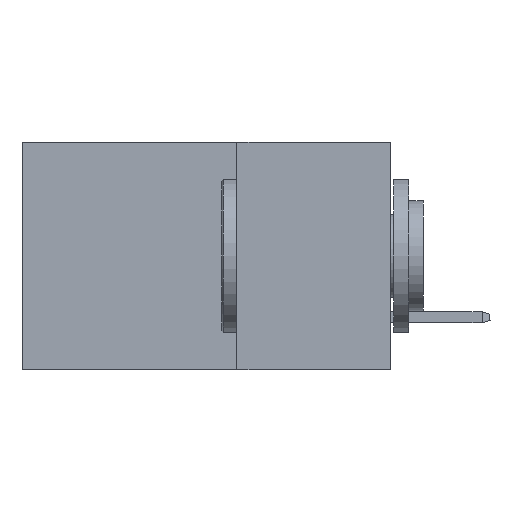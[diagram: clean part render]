
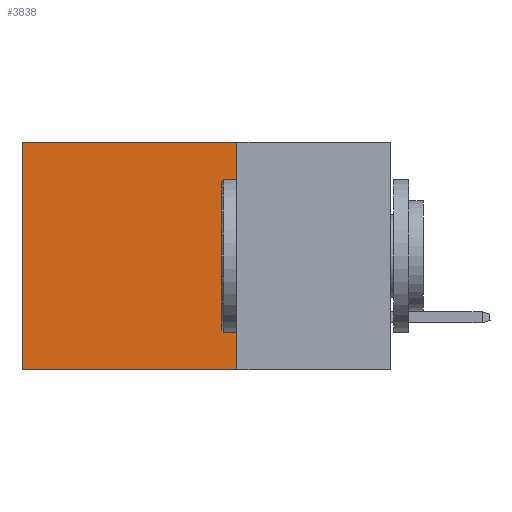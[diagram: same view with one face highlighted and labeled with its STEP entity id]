
A CAD part, left-side view. The second image highlights one B-rep face of the part: STEP entity #3838.
In plain terms, the highlighted planar face has unit normal (-1, 0, 0).
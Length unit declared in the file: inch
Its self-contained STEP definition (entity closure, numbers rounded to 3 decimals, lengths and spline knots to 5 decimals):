
#254 = EDGE_LOOP ( 'NONE', ( #38844, #23494, #27624, #38839 ) ) ;
#633 = CARTESIAN_POINT ( 'NONE',  ( 0.2875, 0.6, 0. ) ) ;
#1068 = DIRECTION ( 'NONE',  ( 0., 1., 0. ) ) ;
#1670 = CARTESIAN_POINT ( 'NONE',  ( 0.2875, 0.6, -0.37 ) ) ;
#3125 = PLANE ( 'NONE',  #3970 ) ;
#3838 = ADVANCED_FACE ( 'NONE', ( #41321 ), #3125, .F. ) ;
#3970 = AXIS2_PLACEMENT_3D ( 'NONE', #22071, #41731, #25519 ) ;
#4987 = LINE ( 'NONE', #633, #29955 ) ;
#8846 = VERTEX_POINT ( 'NONE', #1670 ) ;
#10321 = VECTOR ( 'NONE', #34699, 39.37008 ) ;
#14173 = CARTESIAN_POINT ( 'NONE',  ( 0.2875, 0.6, 0. ) ) ;
#14351 = CARTESIAN_POINT ( 'NONE',  ( 0.2875, 0.25, -0.37 ) ) ;
#15154 = EDGE_CURVE ( 'NONE', #17405, #8846, #37426, .T. ) ;
#15465 = LINE ( 'NONE', #40945, #10321 ) ;
#17405 = VERTEX_POINT ( 'NONE', #14351 ) ;
#19881 = VERTEX_POINT ( 'NONE', #26410 ) ;
#22071 = CARTESIAN_POINT ( 'NONE',  ( 0.2875, 0.25, 0. ) ) ;
#23494 = ORIENTED_EDGE ( 'NONE', *, *, #15154, .F. ) ;
#23806 = EDGE_CURVE ( 'NONE', #36100, #8846, #4987, .T. ) ;
#25519 = DIRECTION ( 'NONE',  ( 0., 0., -1. ) ) ;
#25586 = EDGE_CURVE ( 'NONE', #19881, #36100, #15465, .T. ) ;
#26410 = CARTESIAN_POINT ( 'NONE',  ( 0.2875, 0.25, 0. ) ) ;
#27624 = ORIENTED_EDGE ( 'NONE', *, *, #30389, .F. ) ;
#29955 = VECTOR ( 'NONE', #33783, 39.37008 ) ;
#30389 = EDGE_CURVE ( 'NONE', #19881, #17405, #39308, .T. ) ;
#30665 = VECTOR ( 'NONE', #40249, 39.37008 ) ;
#33783 = DIRECTION ( 'NONE',  ( 0., 0., -1. ) ) ;
#34699 = DIRECTION ( 'NONE',  ( 0., 1., 0. ) ) ;
#36100 = VERTEX_POINT ( 'NONE', #14173 ) ;
#36970 = CARTESIAN_POINT ( 'NONE',  ( 0.2875, 0.25, 0. ) ) ;
#37148 = CARTESIAN_POINT ( 'NONE',  ( 0.2875, 0.25, -0.37 ) ) ;
#37426 = LINE ( 'NONE', #37148, #41003 ) ;
#38839 = ORIENTED_EDGE ( 'NONE', *, *, #25586, .T. ) ;
#38844 = ORIENTED_EDGE ( 'NONE', *, *, #23806, .T. ) ;
#39308 = LINE ( 'NONE', #36970, #30665 ) ;
#40249 = DIRECTION ( 'NONE',  ( 0., 0., -1. ) ) ;
#40945 = CARTESIAN_POINT ( 'NONE',  ( 0.2875, 0.25, 0. ) ) ;
#41003 = VECTOR ( 'NONE', #1068, 39.37008 ) ;
#41321 = FACE_OUTER_BOUND ( 'NONE', #254, .T. ) ;
#41731 = DIRECTION ( 'NONE',  ( 1., 0., 0. ) ) ;
